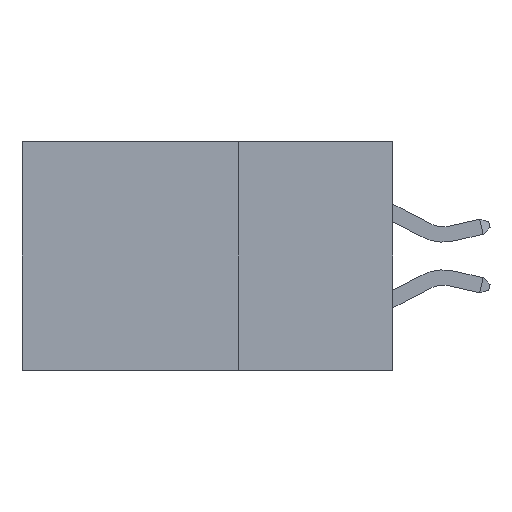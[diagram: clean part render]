
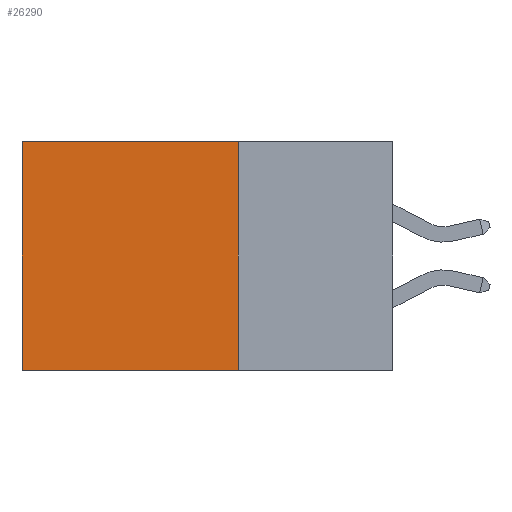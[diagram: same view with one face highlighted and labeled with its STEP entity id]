
A CAD part, left-side view. The second image highlights one B-rep face of the part: STEP entity #26290.
In plain terms, the highlighted planar face has unit normal (-1, 0, 0).
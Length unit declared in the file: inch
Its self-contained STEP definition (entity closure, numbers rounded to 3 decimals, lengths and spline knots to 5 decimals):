
#1068 = DIRECTION ( 'NONE',  ( 0., 1., 0. ) ) ;
#1642 = ORIENTED_EDGE ( 'NONE', *, *, #17807, .T. ) ;
#2100 = LINE ( 'NONE', #17482, #12460 ) ;
#4875 = EDGE_CURVE ( 'NONE', #18481, #9921, #33065, .T. ) ;
#6079 = CARTESIAN_POINT ( 'NONE',  ( 0.2875, 0.6, 0. ) ) ;
#8506 = VERTEX_POINT ( 'NONE', #18264 ) ;
#8675 = AXIS2_PLACEMENT_3D ( 'NONE', #26698, #26822, #26932 ) ;
#8970 = PLANE ( 'NONE',  #8675 ) ;
#9921 = VERTEX_POINT ( 'NONE', #31321 ) ;
#10799 = LINE ( 'NONE', #19385, #21643 ) ;
#10957 = DIRECTION ( 'NONE',  ( 0., 1., 0. ) ) ;
#11316 = DIRECTION ( 'NONE',  ( 0., 0., -1. ) ) ;
#12460 = VECTOR ( 'NONE', #22461, 39.37008 ) ;
#15921 = EDGE_CURVE ( 'NONE', #18481, #8506, #2100, .T. ) ;
#17482 = CARTESIAN_POINT ( 'NONE',  ( 0.2875, 0.25, 0. ) ) ;
#17807 = EDGE_CURVE ( 'NONE', #9921, #23773, #28433, .T. ) ;
#18264 = CARTESIAN_POINT ( 'NONE',  ( 0.2875, 0.25, -0.37 ) ) ;
#18481 = VERTEX_POINT ( 'NONE', #22900 ) ;
#19011 = CARTESIAN_POINT ( 'NONE',  ( 0.2875, 0.25, 0. ) ) ;
#19385 = CARTESIAN_POINT ( 'NONE',  ( 0.2875, 0.25, -0.37 ) ) ;
#21102 = FACE_OUTER_BOUND ( 'NONE', #32207, .T. ) ;
#21181 = VECTOR ( 'NONE', #11316, 39.37008 ) ;
#21643 = VECTOR ( 'NONE', #1068, 39.37008 ) ;
#22461 = DIRECTION ( 'NONE',  ( 0., 0., -1. ) ) ;
#22900 = CARTESIAN_POINT ( 'NONE',  ( 0.2875, 0.25, 0. ) ) ;
#23418 = VECTOR ( 'NONE', #10957, 39.37008 ) ;
#23773 = VERTEX_POINT ( 'NONE', #27071 ) ;
#24523 = ORIENTED_EDGE ( 'NONE', *, *, #15921, .F. ) ;
#26290 = ADVANCED_FACE ( 'NONE', ( #21102 ), #8970, .F. ) ;
#26698 = CARTESIAN_POINT ( 'NONE',  ( 0.2875, 0.25, 0. ) ) ;
#26822 = DIRECTION ( 'NONE',  ( 1., 0., 0. ) ) ;
#26921 = ORIENTED_EDGE ( 'NONE', *, *, #4875, .T. ) ;
#26932 = DIRECTION ( 'NONE',  ( 0., 0., -1. ) ) ;
#27071 = CARTESIAN_POINT ( 'NONE',  ( 0.2875, 0.6, -0.37 ) ) ;
#28433 = LINE ( 'NONE', #6079, #21181 ) ;
#29487 = EDGE_CURVE ( 'NONE', #8506, #23773, #10799, .T. ) ;
#31321 = CARTESIAN_POINT ( 'NONE',  ( 0.2875, 0.6, 0. ) ) ;
#32207 = EDGE_LOOP ( 'NONE', ( #1642, #32958, #24523, #26921 ) ) ;
#32958 = ORIENTED_EDGE ( 'NONE', *, *, #29487, .F. ) ;
#33065 = LINE ( 'NONE', #19011, #23418 ) ;
